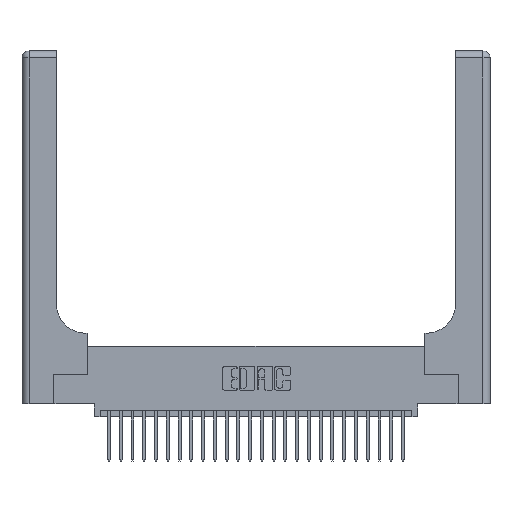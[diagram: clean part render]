
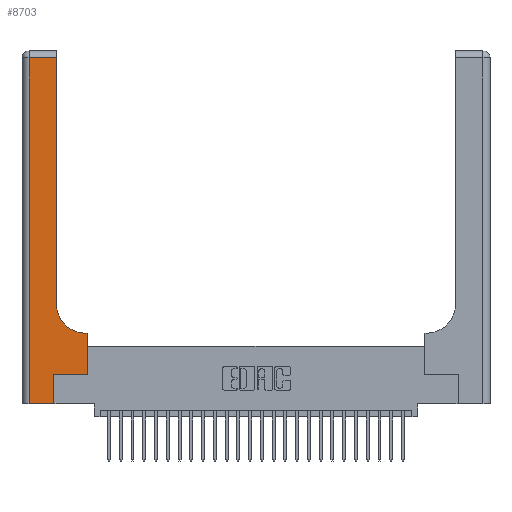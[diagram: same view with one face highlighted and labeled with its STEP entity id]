
A CAD part, top view. The second image highlights one B-rep face of the part: STEP entity #8703.
In plain terms, the highlighted planar face has unit normal (0, 0, 1).
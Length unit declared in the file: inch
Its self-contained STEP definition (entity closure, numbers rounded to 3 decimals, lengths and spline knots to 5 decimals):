
#377 = CARTESIAN_POINT ( 'NONE',  ( 0.2915, 0.85, 0.37 ) ) ;
#741 = EDGE_CURVE ( 'NONE', #15708, #27117, #9962, .T. ) ;
#1510 = CARTESIAN_POINT ( 'NONE',  ( 0.2915, 0.6, 0.37 ) ) ;
#1711 = CARTESIAN_POINT ( 'NONE',  ( 0.5585, 0.25, 0.37 ) ) ;
#1716 = CARTESIAN_POINT ( 'NONE',  ( 0.5415, 0.85, 0.37 ) ) ;
#1740 = EDGE_CURVE ( 'NONE', #10509, #7567, #16664, .T. ) ;
#2663 = EDGE_CURVE ( 'NONE', #27117, #10509, #10217, .T. ) ;
#3222 = LINE ( 'NONE', #26208, #26401 ) ;
#3695 = CARTESIAN_POINT ( 'NONE',  ( 0., 0., 0.37 ) ) ;
#4775 = DIRECTION ( 'NONE',  ( 0., -1., 0. ) ) ;
#4911 = CARTESIAN_POINT ( 'NONE',  ( 0., 3., 0.37 ) ) ;
#5067 = CARTESIAN_POINT ( 'NONE',  ( 0.06, 0., 0.37 ) ) ;
#5144 = ORIENTED_EDGE ( 'NONE', *, *, #26669, .T. ) ;
#5341 = ORIENTED_EDGE ( 'NONE', *, *, #12844, .T. ) ;
#5725 = FACE_OUTER_BOUND ( 'NONE', #6439, .T. ) ;
#5944 = DIRECTION ( 'NONE',  ( 1., 0., 0. ) ) ;
#6439 = EDGE_LOOP ( 'NONE', ( #11057, #5341, #14794, #17818, #16163, #20024, #21486, #12633, #5144 ) ) ;
#7099 = VERTEX_POINT ( 'NONE', #7689 ) ;
#7567 = VERTEX_POINT ( 'NONE', #24158 ) ;
#7689 = CARTESIAN_POINT ( 'NONE',  ( 0.2915, 2.94, 0.37 ) ) ;
#8458 = VERTEX_POINT ( 'NONE', #8532 ) ;
#8532 = CARTESIAN_POINT ( 'NONE',  ( 0.5415, 0.6, 0.37 ) ) ;
#8703 = ADVANCED_FACE ( 'NONE', ( #5725 ), #19864, .F. ) ;
#9962 = LINE ( 'NONE', #26281, #24067 ) ;
#10217 = LINE ( 'NONE', #17839, #21979 ) ;
#10509 = VERTEX_POINT ( 'NONE', #23725 ) ;
#10922 = VECTOR ( 'NONE', #17118, 39.37008 ) ;
#11057 = ORIENTED_EDGE ( 'NONE', *, *, #27578, .T. ) ;
#11117 = DIRECTION ( 'NONE',  ( 0., 1., 0. ) ) ;
#11223 = AXIS2_PLACEMENT_3D ( 'NONE', #1716, #18837, #23151 ) ;
#11381 = DIRECTION ( 'NONE',  ( -1., 0., 0. ) ) ;
#11738 = DIRECTION ( 'NONE',  ( 1., 0., 0. ) ) ;
#12196 = VERTEX_POINT ( 'NONE', #19782 ) ;
#12633 = ORIENTED_EDGE ( 'NONE', *, *, #15270, .T. ) ;
#12844 = EDGE_CURVE ( 'NONE', #7099, #12196, #24984, .T. ) ;
#14493 = VERTEX_POINT ( 'NONE', #377 ) ;
#14794 = ORIENTED_EDGE ( 'NONE', *, *, #16999, .T. ) ;
#15198 = EDGE_CURVE ( 'NONE', #24936, #15708, #21838, .T. ) ;
#15270 = EDGE_CURVE ( 'NONE', #7567, #8458, #23176, .T. ) ;
#15470 = AXIS2_PLACEMENT_3D ( 'NONE', #4911, #22123, #11381 ) ;
#15708 = VERTEX_POINT ( 'NONE', #17933 ) ;
#15902 = CARTESIAN_POINT ( 'NONE',  ( 0.269, 0.25, 0.37 ) ) ;
#16163 = ORIENTED_EDGE ( 'NONE', *, *, #741, .T. ) ;
#16664 = LINE ( 'NONE', #1711, #10922 ) ;
#16999 = EDGE_CURVE ( 'NONE', #12196, #24936, #27520, .T. ) ;
#17118 = DIRECTION ( 'NONE',  ( 0., 1., 0. ) ) ;
#17455 = VECTOR ( 'NONE', #5944, 39.37008 ) ;
#17584 = CIRCLE ( 'NONE', #11223, 0.25 ) ;
#17818 = ORIENTED_EDGE ( 'NONE', *, *, #15198, .T. ) ;
#17839 = CARTESIAN_POINT ( 'NONE',  ( 0.269, 0.25, 0.37 ) ) ;
#17933 = CARTESIAN_POINT ( 'NONE',  ( 0.269, 0., 0.37 ) ) ;
#18837 = DIRECTION ( 'NONE',  ( 0., 0., -1. ) ) ;
#18925 = VECTOR ( 'NONE', #23795, 39.37008 ) ;
#19782 = CARTESIAN_POINT ( 'NONE',  ( 0.06, 2.94, 0.37 ) ) ;
#19864 = PLANE ( 'NONE',  #15470 ) ;
#20024 = ORIENTED_EDGE ( 'NONE', *, *, #2663, .T. ) ;
#21486 = ORIENTED_EDGE ( 'NONE', *, *, #1740, .T. ) ;
#21838 = LINE ( 'NONE', #3695, #17455 ) ;
#21979 = VECTOR ( 'NONE', #11738, 39.37008 ) ;
#22123 = DIRECTION ( 'NONE',  ( 0., 0., -1. ) ) ;
#23151 = DIRECTION ( 'NONE',  ( 1., 0., 0. ) ) ;
#23176 = LINE ( 'NONE', #1510, #27574 ) ;
#23655 = DIRECTION ( 'NONE',  ( 0., 1., 0. ) ) ;
#23725 = CARTESIAN_POINT ( 'NONE',  ( 0.5585, 0.25, 0.37 ) ) ;
#23795 = DIRECTION ( 'NONE',  ( -1., 0., 0. ) ) ;
#23986 = CARTESIAN_POINT ( 'NONE',  ( 0., 2.94, 0.37 ) ) ;
#24067 = VECTOR ( 'NONE', #11117, 39.37008 ) ;
#24101 = VECTOR ( 'NONE', #4775, 39.37008 ) ;
#24158 = CARTESIAN_POINT ( 'NONE',  ( 0.5585, 0.6, 0.37 ) ) ;
#24936 = VERTEX_POINT ( 'NONE', #5067 ) ;
#24984 = LINE ( 'NONE', #23986, #18925 ) ;
#26208 = CARTESIAN_POINT ( 'NONE',  ( 0.2915, 3., 0.37 ) ) ;
#26218 = CARTESIAN_POINT ( 'NONE',  ( 0.06, 3., 0.37 ) ) ;
#26281 = CARTESIAN_POINT ( 'NONE',  ( 0.269, 0., 0.37 ) ) ;
#26401 = VECTOR ( 'NONE', #23655, 39.37008 ) ;
#26669 = EDGE_CURVE ( 'NONE', #8458, #14493, #17584, .T. ) ;
#27117 = VERTEX_POINT ( 'NONE', #15902 ) ;
#27297 = DIRECTION ( 'NONE',  ( -1., 0., 0. ) ) ;
#27520 = LINE ( 'NONE', #26218, #24101 ) ;
#27574 = VECTOR ( 'NONE', #27297, 39.37008 ) ;
#27578 = EDGE_CURVE ( 'NONE', #14493, #7099, #3222, .T. ) ;
